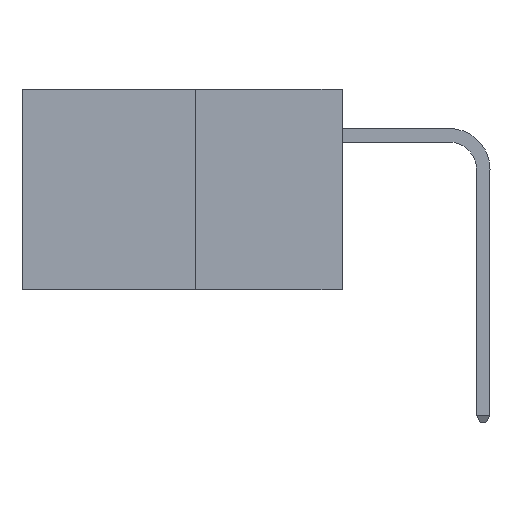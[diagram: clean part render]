
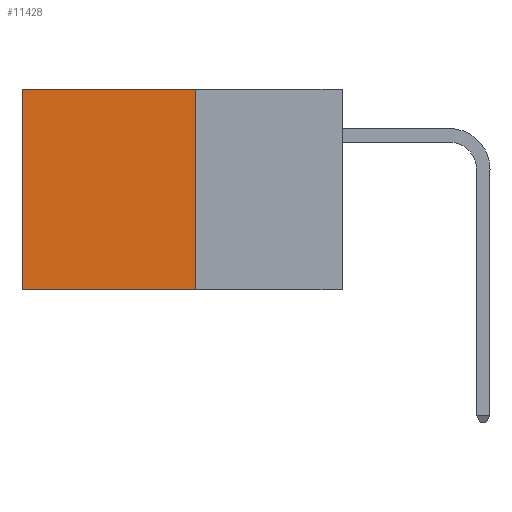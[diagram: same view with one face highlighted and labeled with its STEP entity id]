
A CAD part, left-side view. The second image highlights one B-rep face of the part: STEP entity #11428.
In plain terms, the highlighted planar face has unit normal (-1, 0, 0).
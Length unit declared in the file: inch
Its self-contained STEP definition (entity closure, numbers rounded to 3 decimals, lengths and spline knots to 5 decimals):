
#1018 = VECTOR ( 'NONE', #3780, 39.37008 ) ;
#1681 = CARTESIAN_POINT ( 'NONE',  ( 0.277, 0.27, -0.37 ) ) ;
#2162 = CARTESIAN_POINT ( 'NONE',  ( 0.277, 0.59, -0.37 ) ) ;
#2607 = CARTESIAN_POINT ( 'NONE',  ( 0.277, 0.27, -0.37 ) ) ;
#2859 = VECTOR ( 'NONE', #8745, 39.37008 ) ;
#3780 = DIRECTION ( 'NONE',  ( 0., 0., -1. ) ) ;
#4104 = FACE_OUTER_BOUND ( 'NONE', #18432, .T. ) ;
#4185 = EDGE_CURVE ( 'NONE', #19445, #11581, #15384, .T. ) ;
#5748 = LINE ( 'NONE', #13069, #16676 ) ;
#5851 = DIRECTION ( 'NONE',  ( 1., 0., 0. ) ) ;
#6004 = VERTEX_POINT ( 'NONE', #19486 ) ;
#7532 = ORIENTED_EDGE ( 'NONE', *, *, #13732, .T. ) ;
#8745 = DIRECTION ( 'NONE',  ( 0., 0., -1. ) ) ;
#9928 = CARTESIAN_POINT ( 'NONE',  ( 0.277, 0.27, -0.37 ) ) ;
#10189 = ORIENTED_EDGE ( 'NONE', *, *, #12427, .T. ) ;
#10511 = VERTEX_POINT ( 'NONE', #12774 ) ;
#10668 = ORIENTED_EDGE ( 'NONE', *, *, #11561, .F. ) ;
#11088 = CARTESIAN_POINT ( 'NONE',  ( 0.277, 0.27, -0.37 ) ) ;
#11428 = ADVANCED_FACE ( 'NONE', ( #4104 ), #15176, .F. ) ;
#11561 = EDGE_CURVE ( 'NONE', #11581, #10511, #17279, .T. ) ;
#11581 = VERTEX_POINT ( 'NONE', #1681 ) ;
#12427 = EDGE_CURVE ( 'NONE', #6004, #10511, #13623, .T. ) ;
#12698 = CARTESIAN_POINT ( 'NONE',  ( 0.277, 0.27, 0. ) ) ;
#12774 = CARTESIAN_POINT ( 'NONE',  ( 0.277, 0.59, -0.37 ) ) ;
#13069 = CARTESIAN_POINT ( 'NONE',  ( 0.277, 0.27, 0. ) ) ;
#13178 = VECTOR ( 'NONE', #17334, 39.37008 ) ;
#13623 = LINE ( 'NONE', #2162, #1018 ) ;
#13732 = EDGE_CURVE ( 'NONE', #19445, #6004, #5748, .T. ) ;
#14637 = DIRECTION ( 'NONE',  ( 0., 1., 0. ) ) ;
#15098 = AXIS2_PLACEMENT_3D ( 'NONE', #2607, #5851, #16706 ) ;
#15176 = PLANE ( 'NONE',  #15098 ) ;
#15384 = LINE ( 'NONE', #9928, #2859 ) ;
#16676 = VECTOR ( 'NONE', #14637, 39.37008 ) ;
#16706 = DIRECTION ( 'NONE',  ( 0., 0., -1. ) ) ;
#17279 = LINE ( 'NONE', #11088, #13178 ) ;
#17334 = DIRECTION ( 'NONE',  ( 0., 1., 0. ) ) ;
#18432 = EDGE_LOOP ( 'NONE', ( #10189, #10668, #18967, #7532 ) ) ;
#18967 = ORIENTED_EDGE ( 'NONE', *, *, #4185, .F. ) ;
#19445 = VERTEX_POINT ( 'NONE', #12698 ) ;
#19486 = CARTESIAN_POINT ( 'NONE',  ( 0.277, 0.59, 0. ) ) ;
